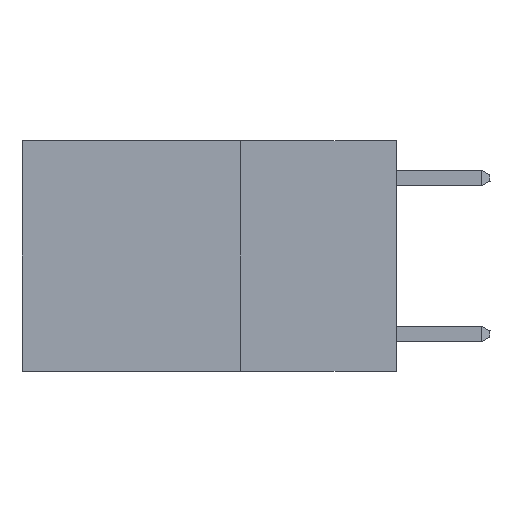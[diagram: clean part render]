
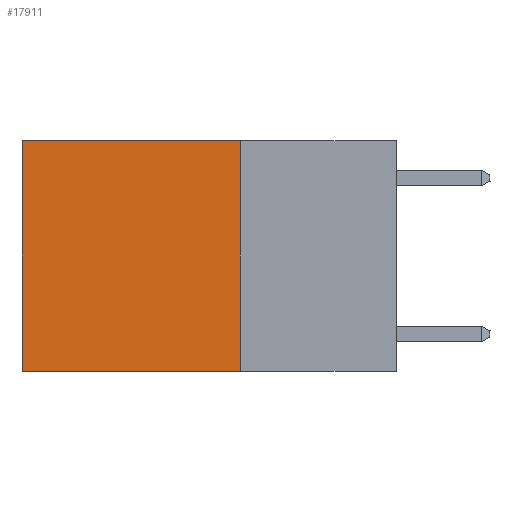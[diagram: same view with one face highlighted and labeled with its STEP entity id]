
A CAD part, left-side view. The second image highlights one B-rep face of the part: STEP entity #17911.
In plain terms, the highlighted planar face has unit normal (-1, 0, 0).
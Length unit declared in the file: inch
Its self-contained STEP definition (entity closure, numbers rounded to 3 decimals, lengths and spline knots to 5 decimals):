
#103 = VECTOR ( 'NONE', #20258, 39.37008 ) ;
#190 = CARTESIAN_POINT ( 'NONE',  ( 0.2625, 0.25, 0. ) ) ;
#503 = PLANE ( 'NONE',  #4158 ) ;
#645 = DIRECTION ( 'NONE',  ( 1., 0., 0. ) ) ;
#889 = VERTEX_POINT ( 'NONE', #9084 ) ;
#3663 = CARTESIAN_POINT ( 'NONE',  ( 0.2625, 0.25, 0. ) ) ;
#4158 = AXIS2_PLACEMENT_3D ( 'NONE', #21010, #645, #20732 ) ;
#4519 = VECTOR ( 'NONE', #11867, 39.37008 ) ;
#6277 = EDGE_CURVE ( 'NONE', #13288, #26024, #12301, .T. ) ;
#7653 = CARTESIAN_POINT ( 'NONE',  ( 0.2625, 0.6, 0. ) ) ;
#8543 = ORIENTED_EDGE ( 'NONE', *, *, #9269, .F. ) ;
#8574 = VECTOR ( 'NONE', #25834, 39.37008 ) ;
#8905 = LINE ( 'NONE', #26910, #103 ) ;
#9084 = CARTESIAN_POINT ( 'NONE',  ( 0.2625, 0.6, -0.37 ) ) ;
#9269 = EDGE_CURVE ( 'NONE', #26024, #889, #8905, .T. ) ;
#11867 = DIRECTION ( 'NONE',  ( 0., 0., -1. ) ) ;
#12257 = CARTESIAN_POINT ( 'NONE',  ( 0.2625, 0.6, 0. ) ) ;
#12301 = LINE ( 'NONE', #23057, #4519 ) ;
#12645 = EDGE_LOOP ( 'NONE', ( #29083, #8543, #26203, #23131 ) ) ;
#13288 = VERTEX_POINT ( 'NONE', #3663 ) ;
#13438 = VERTEX_POINT ( 'NONE', #7653 ) ;
#13651 = LINE ( 'NONE', #190, #19450 ) ;
#14184 = LINE ( 'NONE', #12257, #8574 ) ;
#17349 = CARTESIAN_POINT ( 'NONE',  ( 0.2625, 0.25, -0.37 ) ) ;
#17911 = ADVANCED_FACE ( 'NONE', ( #23224 ), #503, .F. ) ;
#19450 = VECTOR ( 'NONE', #27355, 39.37008 ) ;
#20258 = DIRECTION ( 'NONE',  ( 0., 1., 0. ) ) ;
#20732 = DIRECTION ( 'NONE',  ( 0., 0., -1. ) ) ;
#21010 = CARTESIAN_POINT ( 'NONE',  ( 0.2625, 0.25, 0. ) ) ;
#23057 = CARTESIAN_POINT ( 'NONE',  ( 0.2625, 0.25, 0. ) ) ;
#23131 = ORIENTED_EDGE ( 'NONE', *, *, #26161, .T. ) ;
#23224 = FACE_OUTER_BOUND ( 'NONE', #12645, .T. ) ;
#25432 = EDGE_CURVE ( 'NONE', #13438, #889, #14184, .T. ) ;
#25834 = DIRECTION ( 'NONE',  ( 0., 0., -1. ) ) ;
#26024 = VERTEX_POINT ( 'NONE', #17349 ) ;
#26161 = EDGE_CURVE ( 'NONE', #13288, #13438, #13651, .T. ) ;
#26203 = ORIENTED_EDGE ( 'NONE', *, *, #6277, .F. ) ;
#26910 = CARTESIAN_POINT ( 'NONE',  ( 0.2625, 0.25, -0.37 ) ) ;
#27355 = DIRECTION ( 'NONE',  ( 0., 1., 0. ) ) ;
#29083 = ORIENTED_EDGE ( 'NONE', *, *, #25432, .T. ) ;
